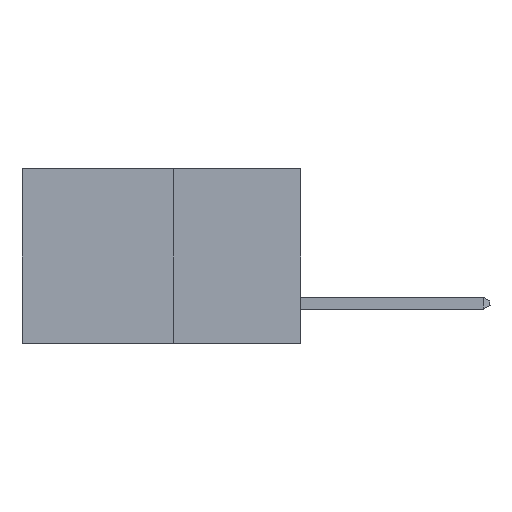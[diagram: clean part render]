
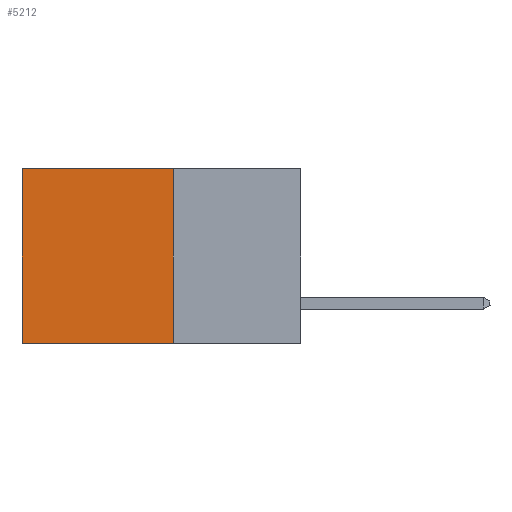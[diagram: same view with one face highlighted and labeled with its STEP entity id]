
A CAD part, left-side view. The second image highlights one B-rep face of the part: STEP entity #5212.
In plain terms, the highlighted planar face has unit normal (-1, 0, 0).
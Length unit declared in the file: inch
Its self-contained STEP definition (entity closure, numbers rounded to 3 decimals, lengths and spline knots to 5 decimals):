
#82 = VECTOR ( 'NONE', #18710, 39.37008 ) ;
#168 = EDGE_CURVE ( 'NONE', #23772, #5097, #4205, .T. ) ;
#331 = CARTESIAN_POINT ( 'NONE',  ( 0.277, 0.59, -0.37 ) ) ;
#3193 = LINE ( 'NONE', #6081, #7876 ) ;
#3643 = ORIENTED_EDGE ( 'NONE', *, *, #22972, .T. ) ;
#4205 = LINE ( 'NONE', #17301, #82 ) ;
#4665 = VECTOR ( 'NONE', #13760, 39.37008 ) ;
#5097 = VERTEX_POINT ( 'NONE', #13675 ) ;
#5212 = ADVANCED_FACE ( 'NONE', ( #10764 ), #9097, .F. ) ;
#5955 = DIRECTION ( 'NONE',  ( 0., 1., 0. ) ) ;
#6081 = CARTESIAN_POINT ( 'NONE',  ( 0.277, 0.27, -0.37 ) ) ;
#6826 = EDGE_CURVE ( 'NONE', #5097, #16318, #3193, .T. ) ;
#7876 = VECTOR ( 'NONE', #5955, 39.37008 ) ;
#8787 = DIRECTION ( 'NONE',  ( 0., 0., -1. ) ) ;
#8816 = DIRECTION ( 'NONE',  ( 1., 0., 0. ) ) ;
#8847 = CARTESIAN_POINT ( 'NONE',  ( 0.277, 0.27, -0.37 ) ) ;
#9097 = PLANE ( 'NONE',  #16322 ) ;
#10764 = FACE_OUTER_BOUND ( 'NONE', #14613, .T. ) ;
#11726 = EDGE_CURVE ( 'NONE', #23772, #23232, #20534, .T. ) ;
#12333 = DIRECTION ( 'NONE',  ( 0., 0., -1. ) ) ;
#13675 = CARTESIAN_POINT ( 'NONE',  ( 0.277, 0.27, -0.37 ) ) ;
#13760 = DIRECTION ( 'NONE',  ( 0., 1., 0. ) ) ;
#14613 = EDGE_LOOP ( 'NONE', ( #3643, #15960, #25035, #24864 ) ) ;
#15190 = CARTESIAN_POINT ( 'NONE',  ( 0.277, 0.27, 0. ) ) ;
#15960 = ORIENTED_EDGE ( 'NONE', *, *, #6826, .F. ) ;
#16318 = VERTEX_POINT ( 'NONE', #21430 ) ;
#16322 = AXIS2_PLACEMENT_3D ( 'NONE', #8847, #8816, #8787 ) ;
#17301 = CARTESIAN_POINT ( 'NONE',  ( 0.277, 0.27, -0.37 ) ) ;
#17419 = CARTESIAN_POINT ( 'NONE',  ( 0.277, 0.59, 0. ) ) ;
#18710 = DIRECTION ( 'NONE',  ( 0., 0., -1. ) ) ;
#20534 = LINE ( 'NONE', #21622, #4665 ) ;
#20952 = VECTOR ( 'NONE', #12333, 39.37008 ) ;
#21430 = CARTESIAN_POINT ( 'NONE',  ( 0.277, 0.59, -0.37 ) ) ;
#21622 = CARTESIAN_POINT ( 'NONE',  ( 0.277, 0.27, 0. ) ) ;
#22183 = LINE ( 'NONE', #331, #20952 ) ;
#22972 = EDGE_CURVE ( 'NONE', #23232, #16318, #22183, .T. ) ;
#23232 = VERTEX_POINT ( 'NONE', #17419 ) ;
#23772 = VERTEX_POINT ( 'NONE', #15190 ) ;
#24864 = ORIENTED_EDGE ( 'NONE', *, *, #11726, .T. ) ;
#25035 = ORIENTED_EDGE ( 'NONE', *, *, #168, .F. ) ;
